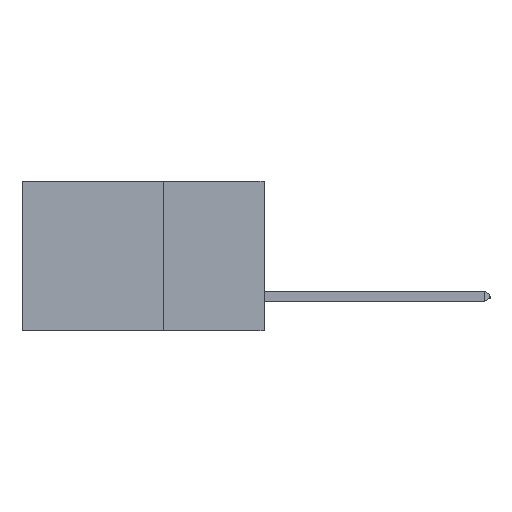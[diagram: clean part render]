
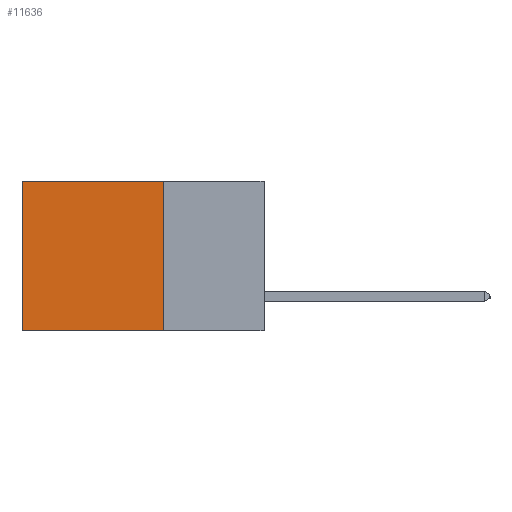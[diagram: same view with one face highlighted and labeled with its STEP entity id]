
A CAD part, left-side view. The second image highlights one B-rep face of the part: STEP entity #11636.
In plain terms, the highlighted planar face has unit normal (-1, 0, 0).
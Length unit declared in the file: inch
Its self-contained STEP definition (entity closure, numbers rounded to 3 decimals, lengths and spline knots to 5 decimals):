
#11 = VERTEX_POINT ( 'NONE', #3463 ) ;
#772 = ORIENTED_EDGE ( 'NONE', *, *, #1723, .T. ) ;
#1067 = VECTOR ( 'NONE', #6884, 39.37008 ) ;
#1356 = VECTOR ( 'NONE', #10026, 39.37008 ) ;
#1723 = EDGE_CURVE ( 'NONE', #4558, #11, #12456, .T. ) ;
#1893 = VERTEX_POINT ( 'NONE', #8026 ) ;
#2640 = VECTOR ( 'NONE', #7499, 39.37008 ) ;
#2920 = CARTESIAN_POINT ( 'NONE',  ( 0.298, 0.25, -0.37 ) ) ;
#3205 = CARTESIAN_POINT ( 'NONE',  ( 0.298, 0.25, 0. ) ) ;
#3279 = PLANE ( 'NONE',  #3500 ) ;
#3463 = CARTESIAN_POINT ( 'NONE',  ( 0.298, 0.6, 0. ) ) ;
#3500 = AXIS2_PLACEMENT_3D ( 'NONE', #6688, #11160, #4448 ) ;
#4448 = DIRECTION ( 'NONE',  ( 0., 0., -1. ) ) ;
#4558 = VERTEX_POINT ( 'NONE', #3205 ) ;
#4865 = FACE_OUTER_BOUND ( 'NONE', #8530, .T. ) ;
#5562 = CARTESIAN_POINT ( 'NONE',  ( 0.298, 0.25, -0.37 ) ) ;
#6067 = LINE ( 'NONE', #9003, #2640 ) ;
#6688 = CARTESIAN_POINT ( 'NONE',  ( 0.298, 0.25, 0. ) ) ;
#6884 = DIRECTION ( 'NONE',  ( 0., 1., 0. ) ) ;
#6936 = CARTESIAN_POINT ( 'NONE',  ( 0.298, 0.25, 0. ) ) ;
#7210 = EDGE_CURVE ( 'NONE', #11, #1893, #6067, .T. ) ;
#7352 = ORIENTED_EDGE ( 'NONE', *, *, #11651, .F. ) ;
#7499 = DIRECTION ( 'NONE',  ( 0., 0., -1. ) ) ;
#7548 = LINE ( 'NONE', #13315, #1356 ) ;
#7798 = VERTEX_POINT ( 'NONE', #5562 ) ;
#8026 = CARTESIAN_POINT ( 'NONE',  ( 0.298, 0.6, -0.37 ) ) ;
#8530 = EDGE_LOOP ( 'NONE', ( #12536, #12309, #7352, #772 ) ) ;
#8647 = DIRECTION ( 'NONE',  ( 0., 1., 0. ) ) ;
#9003 = CARTESIAN_POINT ( 'NONE',  ( 0.298, 0.6, 0. ) ) ;
#10026 = DIRECTION ( 'NONE',  ( 0., 0., -1. ) ) ;
#11160 = DIRECTION ( 'NONE',  ( 1., 0., 0. ) ) ;
#11250 = LINE ( 'NONE', #2920, #13764 ) ;
#11636 = ADVANCED_FACE ( 'NONE', ( #4865 ), #3279, .F. ) ;
#11651 = EDGE_CURVE ( 'NONE', #4558, #7798, #7548, .T. ) ;
#12309 = ORIENTED_EDGE ( 'NONE', *, *, #14018, .F. ) ;
#12456 = LINE ( 'NONE', #6936, #1067 ) ;
#12536 = ORIENTED_EDGE ( 'NONE', *, *, #7210, .T. ) ;
#13315 = CARTESIAN_POINT ( 'NONE',  ( 0.298, 0.25, 0. ) ) ;
#13764 = VECTOR ( 'NONE', #8647, 39.37008 ) ;
#14018 = EDGE_CURVE ( 'NONE', #7798, #1893, #11250, .T. ) ;
